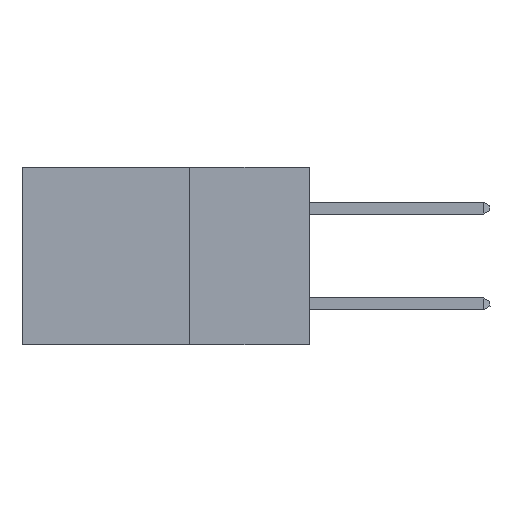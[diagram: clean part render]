
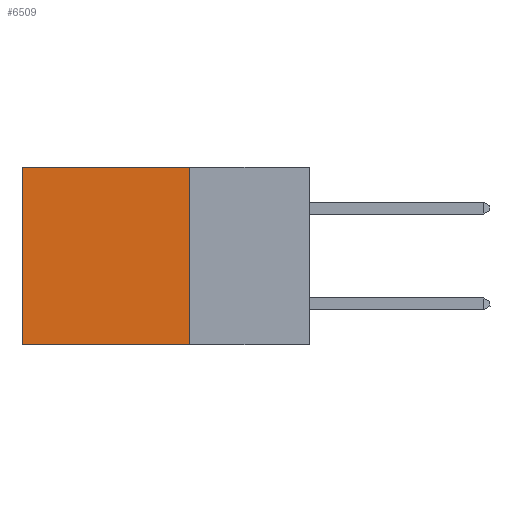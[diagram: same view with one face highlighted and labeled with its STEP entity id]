
A CAD part, left-side view. The second image highlights one B-rep face of the part: STEP entity #6509.
In plain terms, the highlighted planar face has unit normal (-1, 0, 0).
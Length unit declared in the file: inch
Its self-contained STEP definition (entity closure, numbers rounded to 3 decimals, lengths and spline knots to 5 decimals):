
#268 = DIRECTION ( 'NONE',  ( 1., 0., 0. ) ) ;
#358 = VECTOR ( 'NONE', #18301, 39.37008 ) ;
#920 = CARTESIAN_POINT ( 'NONE',  ( 0.2875, 0.6, 0. ) ) ;
#1901 = LINE ( 'NONE', #5294, #16685 ) ;
#2109 = ORIENTED_EDGE ( 'NONE', *, *, #17797, .F. ) ;
#3359 = ORIENTED_EDGE ( 'NONE', *, *, #11857, .T. ) ;
#4232 = CARTESIAN_POINT ( 'NONE',  ( 0.2875, 0.25, 0. ) ) ;
#4345 = AXIS2_PLACEMENT_3D ( 'NONE', #16545, #268, #10578 ) ;
#5139 = CARTESIAN_POINT ( 'NONE',  ( 0.2875, 0.25, 0. ) ) ;
#5294 = CARTESIAN_POINT ( 'NONE',  ( 0.2875, 0.25, -0.37 ) ) ;
#5397 = LINE ( 'NONE', #4232, #12606 ) ;
#5399 = CARTESIAN_POINT ( 'NONE',  ( 0.2875, 0.25, 0. ) ) ;
#5702 = DIRECTION ( 'NONE',  ( 0., 1., 0. ) ) ;
#6150 = VECTOR ( 'NONE', #16631, 39.37008 ) ;
#6368 = CARTESIAN_POINT ( 'NONE',  ( 0.2875, 0.6, 0. ) ) ;
#6509 = ADVANCED_FACE ( 'NONE', ( #6767 ), #13492, .F. ) ;
#6767 = FACE_OUTER_BOUND ( 'NONE', #14073, .T. ) ;
#8984 = EDGE_CURVE ( 'NONE', #12808, #17846, #11630, .T. ) ;
#10578 = DIRECTION ( 'NONE',  ( 0., 0., -1. ) ) ;
#10940 = ORIENTED_EDGE ( 'NONE', *, *, #13442, .T. ) ;
#11164 = VERTEX_POINT ( 'NONE', #19137 ) ;
#11630 = LINE ( 'NONE', #5139, #358 ) ;
#11857 = EDGE_CURVE ( 'NONE', #15326, #11164, #17877, .T. ) ;
#12603 = CARTESIAN_POINT ( 'NONE',  ( 0.2875, 0.25, -0.37 ) ) ;
#12606 = VECTOR ( 'NONE', #5702, 39.37008 ) ;
#12808 = VERTEX_POINT ( 'NONE', #5399 ) ;
#13442 = EDGE_CURVE ( 'NONE', #12808, #15326, #5397, .T. ) ;
#13492 = PLANE ( 'NONE',  #4345 ) ;
#14073 = EDGE_LOOP ( 'NONE', ( #3359, #2109, #14629, #10940 ) ) ;
#14629 = ORIENTED_EDGE ( 'NONE', *, *, #8984, .F. ) ;
#15326 = VERTEX_POINT ( 'NONE', #920 ) ;
#16545 = CARTESIAN_POINT ( 'NONE',  ( 0.2875, 0.25, 0. ) ) ;
#16631 = DIRECTION ( 'NONE',  ( 0., 0., -1. ) ) ;
#16685 = VECTOR ( 'NONE', #18509, 39.37008 ) ;
#17797 = EDGE_CURVE ( 'NONE', #17846, #11164, #1901, .T. ) ;
#17846 = VERTEX_POINT ( 'NONE', #12603 ) ;
#17877 = LINE ( 'NONE', #6368, #6150 ) ;
#18301 = DIRECTION ( 'NONE',  ( 0., 0., -1. ) ) ;
#18509 = DIRECTION ( 'NONE',  ( 0., 1., 0. ) ) ;
#19137 = CARTESIAN_POINT ( 'NONE',  ( 0.2875, 0.6, -0.37 ) ) ;
